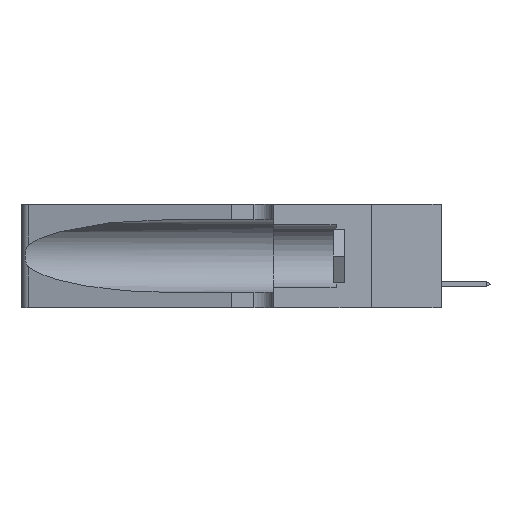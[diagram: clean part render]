
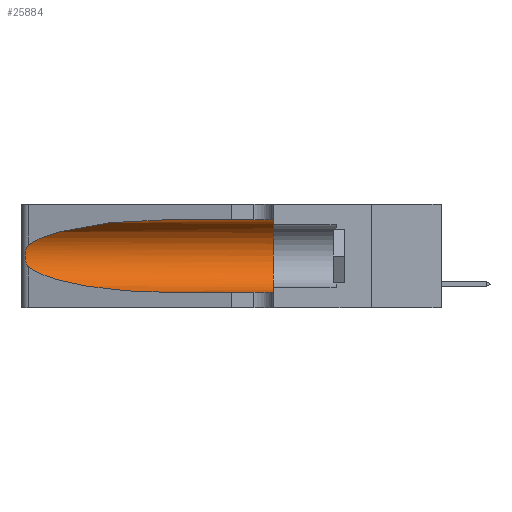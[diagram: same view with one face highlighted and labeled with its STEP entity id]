
A CAD part, left-side view. The second image highlights one B-rep face of the part: STEP entity #25884.
In plain terms, the highlighted cylindrical face has radius 3.308 mm (diameter 6.617 mm), a partial arc.
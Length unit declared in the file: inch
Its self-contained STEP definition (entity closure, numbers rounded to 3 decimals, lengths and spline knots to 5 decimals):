
#79 = DIRECTION ( 'NONE',  ( 0., -1., 0. ) ) ;
#277 = CARTESIAN_POINT ( 'NONE',  ( 0.25487, 1.22718, 0.14631 ) ) ;
#505 = ORIENTED_EDGE ( 'NONE', *, *, #26621, .T. ) ;
#1195 = CARTESIAN_POINT ( 'NONE',  ( 0.25555, 1.22993, 0.14849 ) ) ;
#2231 = AXIS2_PLACEMENT_3D ( 'NONE', #17135, #22261, #14583 ) ;
#2510 = VERTEX_POINT ( 'NONE', #16376 ) ;
#2517 = DIRECTION ( 'NONE',  ( 0., -1., 0. ) ) ;
#3199 = CARTESIAN_POINT ( 'NONE',  ( 0.1305, 0.72297, 0.05475 ) ) ;
#3601 = CARTESIAN_POINT ( 'NONE',  ( 0.26018, 1.23835, 0.19895 ) ) ;
#3728 = EDGE_LOOP ( 'NONE', ( #10953, #16094, #30550, #505, #32101, #8990 ) ) ;
#3819 = VERTEX_POINT ( 'NONE', #22614 ) ;
#4075 = CARTESIAN_POINT ( 'NONE',  ( 0.26075, 1.23896, 0.19203 ) ) ;
#4294 = CYLINDRICAL_SURFACE ( 'NONE', #31647, 0.13025 ) ;
#5134 = DIRECTION ( 'NONE',  ( 0., -1., 0. ) ) ;
#5240 = CARTESIAN_POINT ( 'NONE',  ( 0.1305, 1.61858, 0.31525 ) ) ;
#6632 = EDGE_CURVE ( 'NONE', #26545, #15288, #26389, .T. ) ;
#7628 = CARTESIAN_POINT ( 'NONE',  ( 0.2373, 1.15595, 0.08982 ) ) ;
#8763 = CARTESIAN_POINT ( 'NONE',  ( 0.25856, 1.23593, 0.16098 ) ) ;
#8990 = ORIENTED_EDGE ( 'NONE', *, *, #30116, .F. ) ;
#9424 = EDGE_CURVE ( 'NONE', #26466, #26545, #14224, .T. ) ;
#10953 = ORIENTED_EDGE ( 'NONE', *, *, #32520, .T. ) ;
#11386 = CARTESIAN_POINT ( 'NONE',  ( 0.25639, 1.23186, 0.15144 ) ) ;
#11614 = CARTESIAN_POINT ( 'NONE',  ( 0.25787, 1.23484, 0.2124 ) ) ;
#11795 = LINE ( 'NONE', #5240, #17156 ) ;
#13051 = DIRECTION ( 'NONE',  ( 0., 0., -1. ) ) ;
#14224 = B_SPLINE_CURVE_WITH_KNOTS ( 'NONE', 3,
 ( #19089, #21706, #32661, #11614, #29896, #3601, #4075, #16895, #29674, #8763, #17023, #11386, #1195, #19534 ),
 .UNSPECIFIED., .F., .F.,
 ( 4, 2, 2, 2, 2, 2, 4 ),
 ( 0., 0.00027, 0.00053, 0.00107, 0.0016, 0.00187, 0.00214 ),
 .UNSPECIFIED. ) ;
#14583 = DIRECTION ( 'NONE',  ( 0., 0., 1. ) ) ;
#15288 = VERTEX_POINT ( 'NONE', #3199 ) ;
#16094 = ORIENTED_EDGE ( 'NONE', *, *, #9424, .T. ) ;
#16376 = CARTESIAN_POINT ( 'NONE',  ( 0.1305, 0.72297, 0.31525 ) ) ;
#16895 = CARTESIAN_POINT ( 'NONE',  ( 0.26075, 1.23896, 0.178 ) ) ;
#17023 = CARTESIAN_POINT ( 'NONE',  ( 0.25789, 1.23486, 0.15765 ) ) ;
#17135 = CARTESIAN_POINT ( 'NONE',  ( 0.1305, 0.35, 0.185 ) ) ;
#17156 = VECTOR ( 'NONE', #5134, 39.37008 ) ;
#17418 = CARTESIAN_POINT ( 'NONE',  ( 0.18966, 0.96281, 0.31525 ) ) ;
#19089 = CARTESIAN_POINT ( 'NONE',  ( 0.25487, 1.22718, 0.22369 ) ) ;
#19534 = CARTESIAN_POINT ( 'NONE',  ( 0.25487, 1.22718, 0.14631 ) ) ;
#20146 = CARTESIAN_POINT ( 'NONE',  ( 0.25487, 1.22718, 0.22369 ) ) ;
#20542 = VERTEX_POINT ( 'NONE', #33099 ) ;
#20669 = LINE ( 'NONE', #21041, #24293 ) ;
#21041 = CARTESIAN_POINT ( 'NONE',  ( 0.1305, 1.61858, 0.05475 ) ) ;
#21706 = CARTESIAN_POINT ( 'NONE',  ( 0.25555, 1.22994, 0.2215 ) ) ;
#22261 = DIRECTION ( 'NONE',  ( 0., 1., 0. ) ) ;
#22614 = CARTESIAN_POINT ( 'NONE',  ( 0.1305, 0.35, 0.31525 ) ) ;
#23451 = CARTESIAN_POINT ( 'NONE',  ( 0.1305, 0.72297, 0.05475 ) ) ;
#23547 = FACE_OUTER_BOUND ( 'NONE', #3728, .T. ) ;
#24293 = VECTOR ( 'NONE', #79, 39.37008 ) ;
#24397 = EDGE_CURVE ( 'NONE', #3819, #20542, #28963, .T. ) ;
#25185 = CARTESIAN_POINT ( 'NONE',  ( 0.1305, 0.72297, 0.31525 ) ) ;
#25299 = CARTESIAN_POINT ( 'NONE',  ( 0.2373, 1.15595, 0.28018 ) ) ;
#25884 = ADVANCED_FACE ( 'NONE', ( #23547 ), #4294, .F. ) ;
#25962 = CARTESIAN_POINT ( 'NONE',  ( 0.25487, 1.22718, 0.22369 ) ) ;
#26210 = CARTESIAN_POINT ( 'NONE',  ( 0.1305, 1.61858, 0.185 ) ) ;
#26389 =( BOUNDED_CURVE ( )  B_SPLINE_CURVE ( 3, ( #33587, #7628, #31195, #23451 ),
 .UNSPECIFIED., .F., .F. ) 
 B_SPLINE_CURVE_WITH_KNOTS ( ( 4, 4 ),
 ( 3.44316, 4.71239 ),
 .UNSPECIFIED. ) 
 CURVE ( )  GEOMETRIC_REPRESENTATION_ITEM ( )  RATIONAL_B_SPLINE_CURVE ( ( 1., 0.87, 0.87, 1. ) ) 
 REPRESENTATION_ITEM ( '' )  );
#26466 = VERTEX_POINT ( 'NONE', #25962 ) ;
#26545 = VERTEX_POINT ( 'NONE', #277 ) ;
#26621 = EDGE_CURVE ( 'NONE', #15288, #20542, #20669, .T. ) ;
#28963 = CIRCLE ( 'NONE', #2231, 0.13025 ) ;
#28981 =( BOUNDED_CURVE ( )  B_SPLINE_CURVE ( 3, ( #25185, #17418, #25299, #20146 ),
 .UNSPECIFIED., .F., .F. ) 
 B_SPLINE_CURVE_WITH_KNOTS ( ( 4, 4 ),
 ( 1.5708, 2.84003 ),
 .UNSPECIFIED. ) 
 CURVE ( )  GEOMETRIC_REPRESENTATION_ITEM ( )  RATIONAL_B_SPLINE_CURVE ( ( 1., 0.87, 0.87, 1. ) ) 
 REPRESENTATION_ITEM ( '' )  );
#29674 = CARTESIAN_POINT ( 'NONE',  ( 0.26017, 1.23833, 0.17102 ) ) ;
#29896 = CARTESIAN_POINT ( 'NONE',  ( 0.25854, 1.2359, 0.20912 ) ) ;
#30116 = EDGE_CURVE ( 'NONE', #2510, #3819, #11795, .T. ) ;
#30550 = ORIENTED_EDGE ( 'NONE', *, *, #6632, .T. ) ;
#31195 = CARTESIAN_POINT ( 'NONE',  ( 0.18966, 0.96281, 0.05475 ) ) ;
#31647 = AXIS2_PLACEMENT_3D ( 'NONE', #26210, #2517, #13051 ) ;
#32101 = ORIENTED_EDGE ( 'NONE', *, *, #24397, .F. ) ;
#32520 = EDGE_CURVE ( 'NONE', #2510, #26466, #28981, .T. ) ;
#32661 = CARTESIAN_POINT ( 'NONE',  ( 0.25639, 1.23184, 0.21858 ) ) ;
#33099 = CARTESIAN_POINT ( 'NONE',  ( 0.1305, 0.35, 0.05475 ) ) ;
#33587 = CARTESIAN_POINT ( 'NONE',  ( 0.25487, 1.22718, 0.14631 ) ) ;
